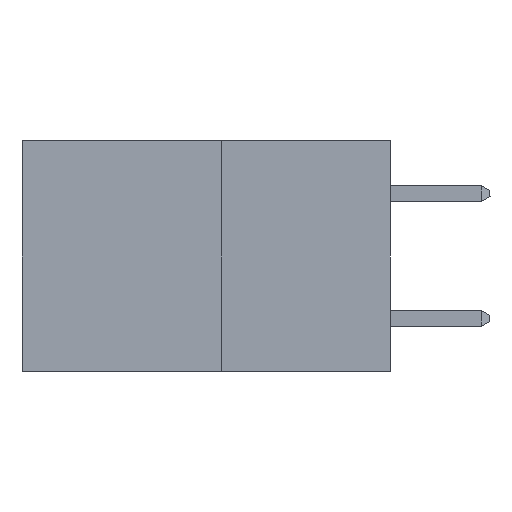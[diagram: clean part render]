
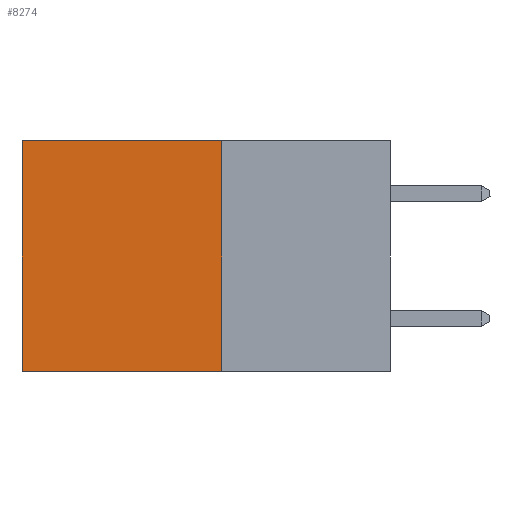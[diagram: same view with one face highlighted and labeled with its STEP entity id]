
A CAD part, left-side view. The second image highlights one B-rep face of the part: STEP entity #8274.
In plain terms, the highlighted planar face has unit normal (-1, 0, 0).
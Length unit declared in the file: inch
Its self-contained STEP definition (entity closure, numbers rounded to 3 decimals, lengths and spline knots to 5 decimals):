
#1113 = FACE_OUTER_BOUND ( 'NONE', #19057, .T. ) ;
#1997 = VECTOR ( 'NONE', #14893, 39.37008 ) ;
#3108 = ORIENTED_EDGE ( 'NONE', *, *, #33513, .F. ) ;
#4041 = CARTESIAN_POINT ( 'NONE',  ( 0.277, 0.27, -0.37 ) ) ;
#5646 = CARTESIAN_POINT ( 'NONE',  ( 0.277, 0.27, -0.37 ) ) ;
#6237 = ORIENTED_EDGE ( 'NONE', *, *, #19757, .F. ) ;
#6658 = DIRECTION ( 'NONE',  ( 0., 0., -1. ) ) ;
#7496 = VERTEX_POINT ( 'NONE', #11545 ) ;
#7928 = VECTOR ( 'NONE', #8362, 39.37008 ) ;
#8274 = ADVANCED_FACE ( 'NONE', ( #1113 ), #11511, .F. ) ;
#8362 = DIRECTION ( 'NONE',  ( 0., 1., 0. ) ) ;
#10409 = EDGE_CURVE ( 'NONE', #14767, #22497, #18164, .T. ) ;
#11511 = PLANE ( 'NONE',  #15843 ) ;
#11545 = CARTESIAN_POINT ( 'NONE',  ( 0.277, 0.59, -0.37 ) ) ;
#11952 = VECTOR ( 'NONE', #17568, 39.37008 ) ;
#14155 = DIRECTION ( 'NONE',  ( 0., 0., -1. ) ) ;
#14767 = VERTEX_POINT ( 'NONE', #22625 ) ;
#14893 = DIRECTION ( 'NONE',  ( 0., 0., -1. ) ) ;
#15843 = AXIS2_PLACEMENT_3D ( 'NONE', #19406, #30164, #14155 ) ;
#17568 = DIRECTION ( 'NONE',  ( 0., 1., 0. ) ) ;
#18164 = LINE ( 'NONE', #25534, #11952 ) ;
#18772 = LINE ( 'NONE', #4041, #31344 ) ;
#19057 = EDGE_LOOP ( 'NONE', ( #22890, #3108, #6237, #28563 ) ) ;
#19406 = CARTESIAN_POINT ( 'NONE',  ( 0.277, 0.27, -0.37 ) ) ;
#19757 = EDGE_CURVE ( 'NONE', #14767, #25181, #18772, .T. ) ;
#19806 = EDGE_CURVE ( 'NONE', #22497, #7496, #24192, .T. ) ;
#21377 = CARTESIAN_POINT ( 'NONE',  ( 0.277, 0.59, 0. ) ) ;
#22497 = VERTEX_POINT ( 'NONE', #21377 ) ;
#22625 = CARTESIAN_POINT ( 'NONE',  ( 0.277, 0.27, 0. ) ) ;
#22847 = CARTESIAN_POINT ( 'NONE',  ( 0.277, 0.59, -0.37 ) ) ;
#22890 = ORIENTED_EDGE ( 'NONE', *, *, #19806, .T. ) ;
#24192 = LINE ( 'NONE', #22847, #1997 ) ;
#25181 = VERTEX_POINT ( 'NONE', #31634 ) ;
#25534 = CARTESIAN_POINT ( 'NONE',  ( 0.277, 0.27, 0. ) ) ;
#28563 = ORIENTED_EDGE ( 'NONE', *, *, #10409, .T. ) ;
#29176 = LINE ( 'NONE', #5646, #7928 ) ;
#30164 = DIRECTION ( 'NONE',  ( 1., 0., 0. ) ) ;
#31344 = VECTOR ( 'NONE', #6658, 39.37008 ) ;
#31634 = CARTESIAN_POINT ( 'NONE',  ( 0.277, 0.27, -0.37 ) ) ;
#33513 = EDGE_CURVE ( 'NONE', #25181, #7496, #29176, .T. ) ;
